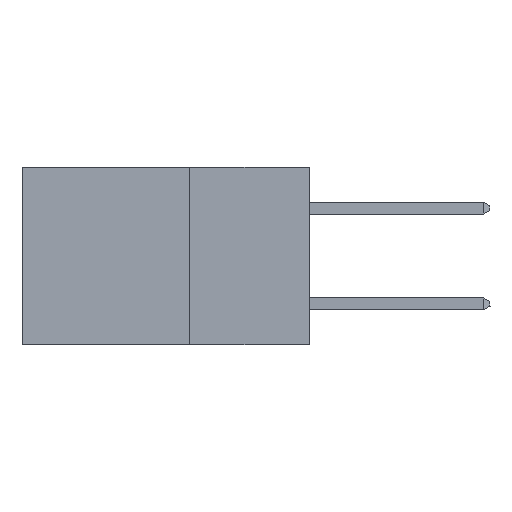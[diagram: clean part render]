
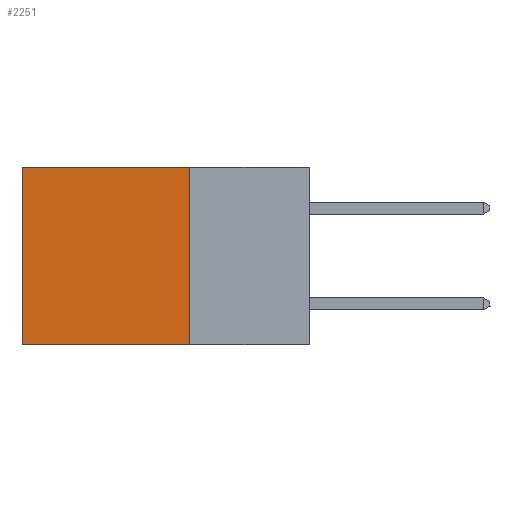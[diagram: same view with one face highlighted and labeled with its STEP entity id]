
A CAD part, left-side view. The second image highlights one B-rep face of the part: STEP entity #2251.
In plain terms, the highlighted planar face has unit normal (-1, 0, 0).
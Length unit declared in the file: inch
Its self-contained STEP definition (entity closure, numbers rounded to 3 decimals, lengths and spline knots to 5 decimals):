
#14 = ORIENTED_EDGE ( 'NONE', *, *, #20543, .F. ) ;
#845 = DIRECTION ( 'NONE',  ( 0., 1., 0. ) ) ;
#2010 = LINE ( 'NONE', #6416, #14835 ) ;
#2251 = ADVANCED_FACE ( 'NONE', ( #5801 ), #6538, .F. ) ;
#3416 = LINE ( 'NONE', #6086, #18337 ) ;
#3907 = VECTOR ( 'NONE', #845, 39.37008 ) ;
#4408 = DIRECTION ( 'NONE',  ( 0., 0., -1. ) ) ;
#4762 = DIRECTION ( 'NONE',  ( 0., 0., -1. ) ) ;
#5059 = CARTESIAN_POINT ( 'NONE',  ( 0.2875, 0.6, -0.37 ) ) ;
#5316 = CARTESIAN_POINT ( 'NONE',  ( 0.2875, 0.25, -0.37 ) ) ;
#5745 = ORIENTED_EDGE ( 'NONE', *, *, #13732, .T. ) ;
#5801 = FACE_OUTER_BOUND ( 'NONE', #12548, .T. ) ;
#5911 = CARTESIAN_POINT ( 'NONE',  ( 0.2875, 0.25, 0. ) ) ;
#6086 = CARTESIAN_POINT ( 'NONE',  ( 0.2875, 0.25, 0. ) ) ;
#6416 = CARTESIAN_POINT ( 'NONE',  ( 0.2875, 0.25, -0.37 ) ) ;
#6538 = PLANE ( 'NONE',  #13607 ) ;
#6945 = LINE ( 'NONE', #10264, #3907 ) ;
#7985 = DIRECTION ( 'NONE',  ( 0., 1., 0. ) ) ;
#9245 = EDGE_CURVE ( 'NONE', #20869, #17038, #15305, .T. ) ;
#9731 = CARTESIAN_POINT ( 'NONE',  ( 0.2875, 0.25, 0. ) ) ;
#9819 = ORIENTED_EDGE ( 'NONE', *, *, #18298, .F. ) ;
#10264 = CARTESIAN_POINT ( 'NONE',  ( 0.2875, 0.25, 0. ) ) ;
#12548 = EDGE_LOOP ( 'NONE', ( #19095, #9819, #14, #5745 ) ) ;
#13607 = AXIS2_PLACEMENT_3D ( 'NONE', #9731, #19425, #4762 ) ;
#13732 = EDGE_CURVE ( 'NONE', #20929, #20869, #6945, .T. ) ;
#14272 = DIRECTION ( 'NONE',  ( 0., 0., -1. ) ) ;
#14835 = VECTOR ( 'NONE', #7985, 39.37008 ) ;
#15036 = VECTOR ( 'NONE', #4408, 39.37008 ) ;
#15305 = LINE ( 'NONE', #16094, #15036 ) ;
#16094 = CARTESIAN_POINT ( 'NONE',  ( 0.2875, 0.6, 0. ) ) ;
#17038 = VERTEX_POINT ( 'NONE', #5059 ) ;
#17079 = CARTESIAN_POINT ( 'NONE',  ( 0.2875, 0.6, 0. ) ) ;
#18298 = EDGE_CURVE ( 'NONE', #19032, #17038, #2010, .T. ) ;
#18337 = VECTOR ( 'NONE', #14272, 39.37008 ) ;
#19032 = VERTEX_POINT ( 'NONE', #5316 ) ;
#19095 = ORIENTED_EDGE ( 'NONE', *, *, #9245, .T. ) ;
#19425 = DIRECTION ( 'NONE',  ( 1., 0., 0. ) ) ;
#20543 = EDGE_CURVE ( 'NONE', #20929, #19032, #3416, .T. ) ;
#20869 = VERTEX_POINT ( 'NONE', #17079 ) ;
#20929 = VERTEX_POINT ( 'NONE', #5911 ) ;
